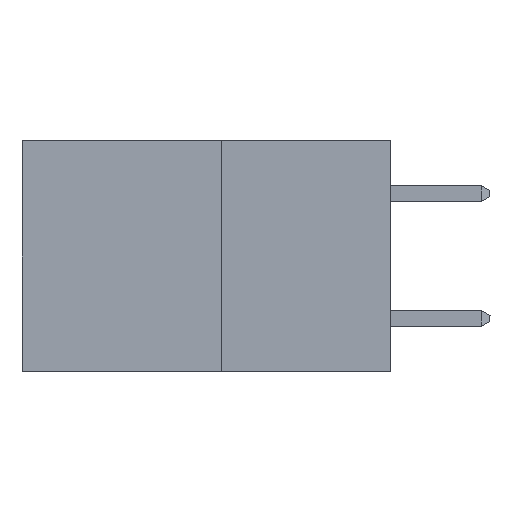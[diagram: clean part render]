
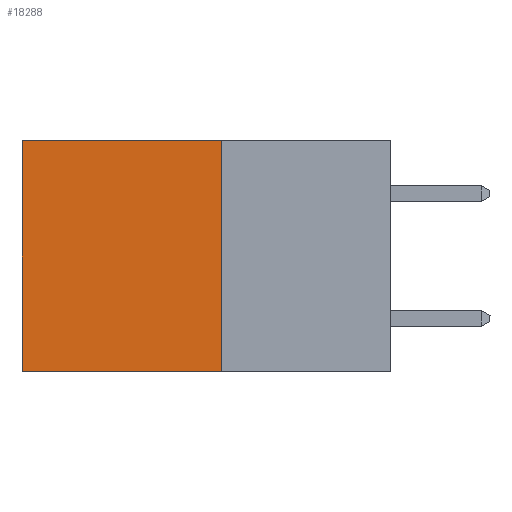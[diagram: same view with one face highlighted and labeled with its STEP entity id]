
A CAD part, left-side view. The second image highlights one B-rep face of the part: STEP entity #18288.
In plain terms, the highlighted planar face has unit normal (-1, 0, 0).
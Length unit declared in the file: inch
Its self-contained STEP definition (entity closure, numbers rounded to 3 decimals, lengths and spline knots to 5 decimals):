
#553 = LINE ( 'NONE', #4871, #15466 ) ;
#2918 = FACE_OUTER_BOUND ( 'NONE', #25304, .T. ) ;
#3979 = LINE ( 'NONE', #14058, #9636 ) ;
#4871 = CARTESIAN_POINT ( 'NONE',  ( 0.277, 0.27, -0.37 ) ) ;
#5193 = PLANE ( 'NONE',  #31217 ) ;
#7022 = ORIENTED_EDGE ( 'NONE', *, *, #26498, .F. ) ;
#7584 = VERTEX_POINT ( 'NONE', #33708 ) ;
#7815 = CARTESIAN_POINT ( 'NONE',  ( 0.277, 0.59, -0.37 ) ) ;
#8480 = DIRECTION ( 'NONE',  ( 0., 0., -1. ) ) ;
#9636 = VECTOR ( 'NONE', #8480, 39.37008 ) ;
#10026 = VERTEX_POINT ( 'NONE', #7815 ) ;
#10379 = CARTESIAN_POINT ( 'NONE',  ( 0.277, 0.59, -0.37 ) ) ;
#10856 = DIRECTION ( 'NONE',  ( 0., 0., -1. ) ) ;
#12394 = CARTESIAN_POINT ( 'NONE',  ( 0.277, 0.27, 0. ) ) ;
#13494 = EDGE_CURVE ( 'NONE', #35451, #15856, #3979, .T. ) ;
#14058 = CARTESIAN_POINT ( 'NONE',  ( 0.277, 0.27, -0.37 ) ) ;
#14774 = LINE ( 'NONE', #10379, #29435 ) ;
#15172 = LINE ( 'NONE', #12394, #24281 ) ;
#15466 = VECTOR ( 'NONE', #21602, 39.37008 ) ;
#15856 = VERTEX_POINT ( 'NONE', #27730 ) ;
#16072 = ORIENTED_EDGE ( 'NONE', *, *, #28115, .T. ) ;
#17962 = DIRECTION ( 'NONE',  ( 0., 1., 0. ) ) ;
#18288 = ADVANCED_FACE ( 'NONE', ( #2918 ), #5193, .F. ) ;
#20943 = ORIENTED_EDGE ( 'NONE', *, *, #13494, .F. ) ;
#21478 = DIRECTION ( 'NONE',  ( 0., 0., -1. ) ) ;
#21602 = DIRECTION ( 'NONE',  ( 0., 1., 0. ) ) ;
#24281 = VECTOR ( 'NONE', #17962, 39.37008 ) ;
#24711 = CARTESIAN_POINT ( 'NONE',  ( 0.277, 0.27, -0.37 ) ) ;
#25304 = EDGE_LOOP ( 'NONE', ( #35154, #7022, #20943, #16072 ) ) ;
#26498 = EDGE_CURVE ( 'NONE', #15856, #10026, #553, .T. ) ;
#27460 = DIRECTION ( 'NONE',  ( 1., 0., 0. ) ) ;
#27730 = CARTESIAN_POINT ( 'NONE',  ( 0.277, 0.27, -0.37 ) ) ;
#28115 = EDGE_CURVE ( 'NONE', #35451, #7584, #15172, .T. ) ;
#29435 = VECTOR ( 'NONE', #21478, 39.37008 ) ;
#30014 = CARTESIAN_POINT ( 'NONE',  ( 0.277, 0.27, 0. ) ) ;
#31217 = AXIS2_PLACEMENT_3D ( 'NONE', #24711, #27460, #10856 ) ;
#33708 = CARTESIAN_POINT ( 'NONE',  ( 0.277, 0.59, 0. ) ) ;
#34011 = EDGE_CURVE ( 'NONE', #7584, #10026, #14774, .T. ) ;
#35154 = ORIENTED_EDGE ( 'NONE', *, *, #34011, .T. ) ;
#35451 = VERTEX_POINT ( 'NONE', #30014 ) ;
